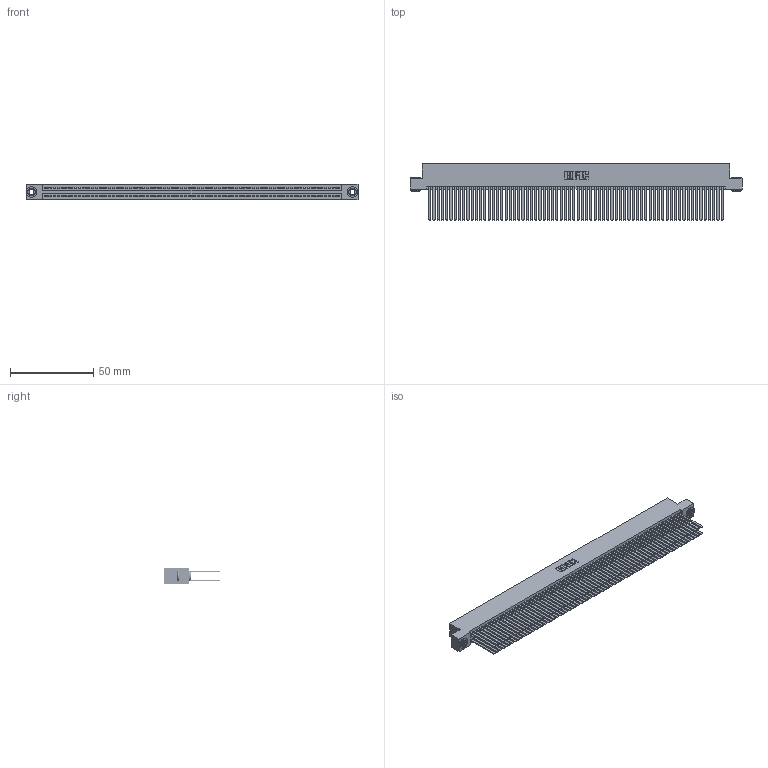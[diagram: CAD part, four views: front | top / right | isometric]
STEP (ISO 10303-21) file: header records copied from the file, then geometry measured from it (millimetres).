
FILE_DESCRIPTION (( 'STEP AP203' ), '1' );
FILE_NAME ('395-140-544-203.STEP', '2019-10-30T01:55:47', ( '' ), ( '' ), 'SwSTEP 2.0', 'SolidWorks 2016', '' );
FILE_SCHEMA (( 'CONFIG_CONTROL_DESIGN' ));
Length unit declared in the file: inch
Products named in the file (4): 345-292-001_345-293-144; 345-250-002_345-250-002-102; 395-140-544-203; 345 Part_Flush Mounting Lugs - 0.156 Dia-TH
Assembly tree (143 placements, depth 2):
  395-140-544-203
    345 Part_Flush Mounting Lugs - 0.156 Dia-TH
    345-292-001_345-293-144  x140
    345-250-002_345-250-002-102  x2
Bounding box: 199.01 x 33.96 x 9.4 mm (x, y, z)
Volume: 21573.8 mm3; surface area: 38388.9 mm2
Topology: 143 solids, 143 shells, 6324 faces, 18757 edges, 12314 vertices
Faces by surface type: plane 4150, cylinder 2166, cone 8
Entity records: 51620 total; most frequent: CARTESIAN_POINT 8599, ORIENTED_EDGE 8526, DIRECTION 7577, EDGE_CURVE 4263, LINE 3831, VECTOR 3831, VERTEX_POINT 2838, AXIS2_PLACEMENT_3D 1873
